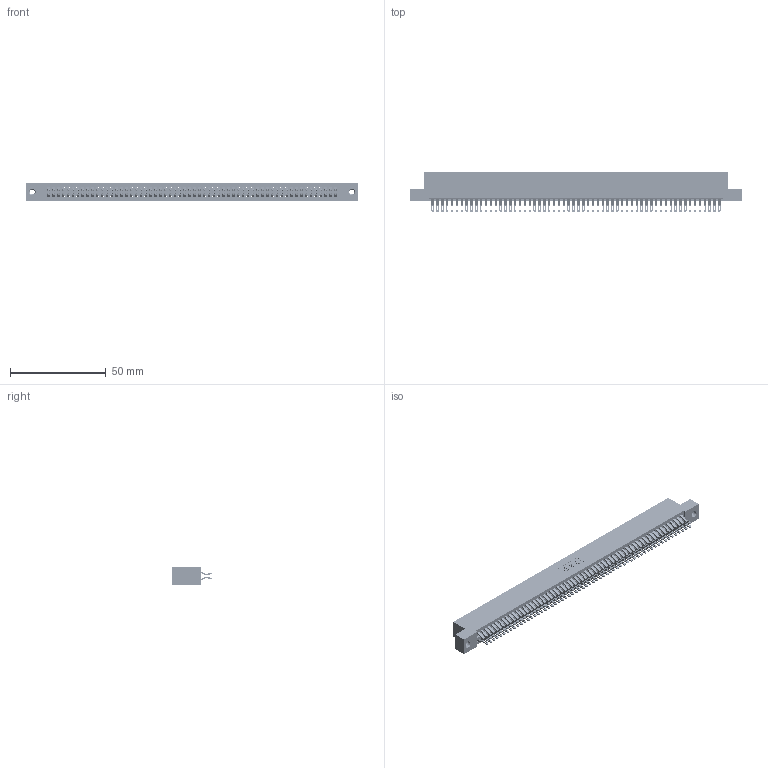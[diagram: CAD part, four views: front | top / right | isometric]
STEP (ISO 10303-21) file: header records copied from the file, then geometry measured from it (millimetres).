
FILE_DESCRIPTION (( 'STEP AP203' ), '1' );
FILE_NAME ('345-120-555-207.STEP', '2019-11-06T03:05:33', ( '' ), ( '' ), 'SwSTEP 2.0', 'SolidWorks 2016', '' );
FILE_SCHEMA (( 'CONFIG_CONTROL_DESIGN' ));
Length unit declared in the file: inch
Products named in the file (4): 345-250-001_345-250-005-103; 345-292-001_555 Tail; 345 Part_Flush Mounting Lugs - 0.156 Dia-TI; 345-120-555-207
Assembly tree (123 placements, depth 2):
  345-120-555-207
    345 Part_Flush Mounting Lugs - 0.156 Dia-TI
    345-292-001_555 Tail  x120
    345-250-001_345-250-005-103  x2
Bounding box: 173.61 x 21.13 x 9.4 mm (x, y, z)
Volume: 17366.2 mm3; surface area: 27257.3 mm2
Topology: 123 solids, 123 shells, 6906 faces, 21717 edges, 14470 vertices
Faces by surface type: plane 3832, cylinder 3058, cone 12, torus 4
Entity records: 46166 total; most frequent: CARTESIAN_POINT 7737, ORIENTED_EDGE 7634, DIRECTION 6795, EDGE_CURVE 3817, LINE 3405, VECTOR 3405, VERTEX_POINT 2540, AXIS2_PLACEMENT_3D 1695
